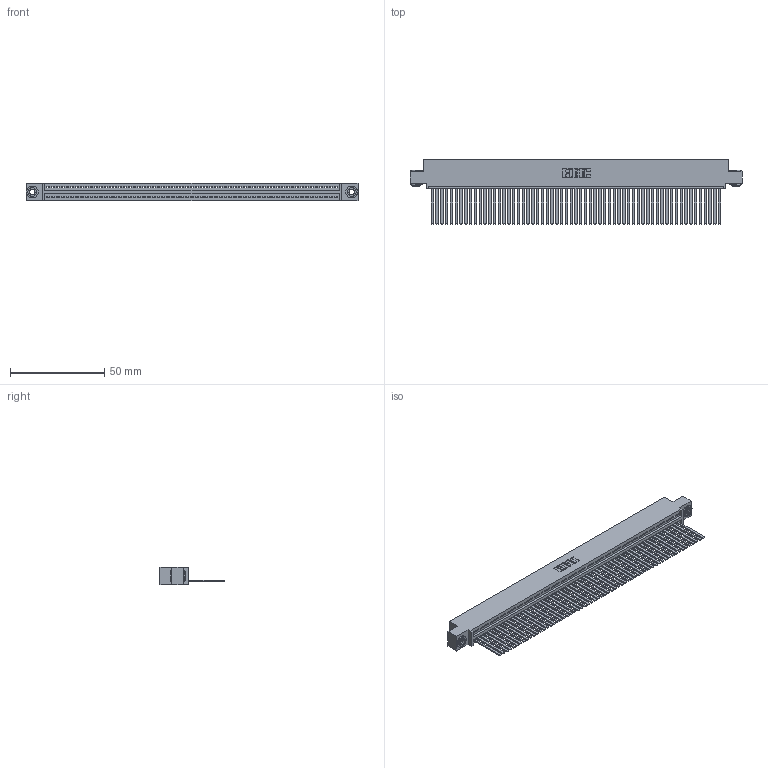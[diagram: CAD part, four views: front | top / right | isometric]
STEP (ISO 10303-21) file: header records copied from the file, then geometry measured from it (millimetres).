
FILE_DESCRIPTION (( 'STEP AP203' ), '1' );
FILE_NAME ('345-061-544-403.STEP', '2019-10-11T03:26:20', ( '' ), ( '' ), 'SwSTEP 2.0', 'SolidWorks 2016', '' );
FILE_SCHEMA (( 'CONFIG_CONTROL_DESIGN' ));
Length unit declared in the file: inch
Products named in the file (4): 345-061-544-403; 345 Part_0.110 Offset - 0.156 Dia-TH; 345-292-001_345-293-144; 345-250-002_345-250-002-102
Assembly tree (64 placements, depth 2):
  345-061-544-403
    345 Part_0.110 Offset - 0.156 Dia-TH
    345-292-001_345-293-144  x61
    345-250-002_345-250-002-102  x2
Bounding box: 176.15 x 33.96 x 9.4 mm (x, y, z)
Volume: 17538.9 mm3; surface area: 25983.1 mm2
Topology: 64 solids, 64 shells, 3340 faces, 10067 edges, 6626 vertices
Faces by surface type: plane 2290, cylinder 1042, cone 8
Entity records: 43950 total; most frequent: CARTESIAN_POINT 7590, ORIENTED_EDGE 7578, DIRECTION 6629, EDGE_CURVE 3789, VECTOR 3393, LINE 3393, VERTEX_POINT 2522, AXIS2_PLACEMENT_3D 1618
